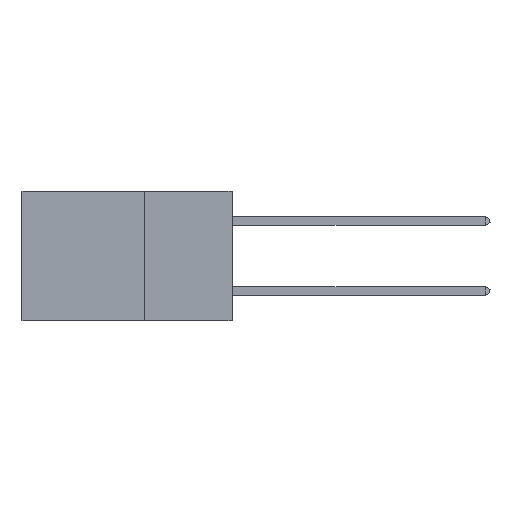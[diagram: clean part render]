
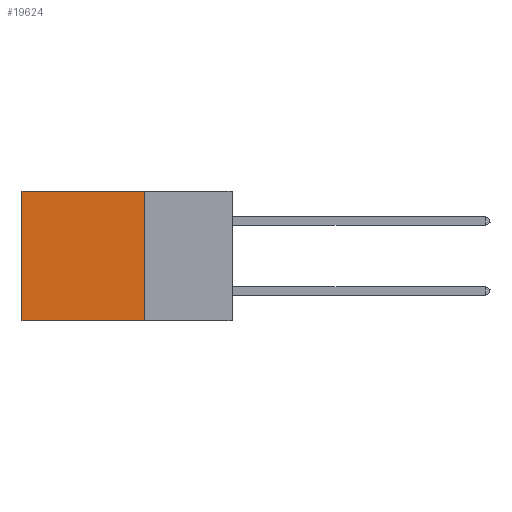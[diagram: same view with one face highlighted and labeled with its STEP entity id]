
A CAD part, left-side view. The second image highlights one B-rep face of the part: STEP entity #19624.
In plain terms, the highlighted planar face has unit normal (-1, 0, 0).
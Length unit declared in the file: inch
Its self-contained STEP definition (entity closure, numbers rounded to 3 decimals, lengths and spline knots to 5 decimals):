
#55 = EDGE_CURVE ( 'NONE', #11595, #7281, #10687, .T. ) ;
#1050 = ORIENTED_EDGE ( 'NONE', *, *, #6455, .F. ) ;
#1164 = CARTESIAN_POINT ( 'NONE',  ( 0.2875, 0.25, -0.37 ) ) ;
#1235 = CARTESIAN_POINT ( 'NONE',  ( 0.2875, 0.6, 0. ) ) ;
#1429 = ORIENTED_EDGE ( 'NONE', *, *, #4409, .T. ) ;
#2161 = ORIENTED_EDGE ( 'NONE', *, *, #55, .T. ) ;
#2571 = LINE ( 'NONE', #23844, #16280 ) ;
#2996 = CARTESIAN_POINT ( 'NONE',  ( 0.2875, 0.6, 0. ) ) ;
#3052 = DIRECTION ( 'NONE',  ( 0., 0., -1. ) ) ;
#4409 = EDGE_CURVE ( 'NONE', #7281, #14466, #6045, .T. ) ;
#4713 = DIRECTION ( 'NONE',  ( 0., 0., -1. ) ) ;
#5467 = VERTEX_POINT ( 'NONE', #1164 ) ;
#5556 = LINE ( 'NONE', #22024, #10125 ) ;
#6045 = LINE ( 'NONE', #2996, #20780 ) ;
#6455 = EDGE_CURVE ( 'NONE', #11595, #5467, #2571, .T. ) ;
#7241 = DIRECTION ( 'NONE',  ( 1., 0., 0. ) ) ;
#7281 = VERTEX_POINT ( 'NONE', #1235 ) ;
#8701 = ORIENTED_EDGE ( 'NONE', *, *, #15763, .F. ) ;
#10125 = VECTOR ( 'NONE', #12718, 39.37008 ) ;
#10687 = LINE ( 'NONE', #15584, #15217 ) ;
#11054 = CARTESIAN_POINT ( 'NONE',  ( 0.2875, 0.25, 0. ) ) ;
#11595 = VERTEX_POINT ( 'NONE', #11054 ) ;
#12066 = EDGE_LOOP ( 'NONE', ( #1429, #8701, #1050, #2161 ) ) ;
#12718 = DIRECTION ( 'NONE',  ( 0., 1., 0. ) ) ;
#14466 = VERTEX_POINT ( 'NONE', #19636 ) ;
#15217 = VECTOR ( 'NONE', #23816, 39.37008 ) ;
#15584 = CARTESIAN_POINT ( 'NONE',  ( 0.2875, 0.25, 0. ) ) ;
#15625 = AXIS2_PLACEMENT_3D ( 'NONE', #18751, #7241, #20661 ) ;
#15657 = FACE_OUTER_BOUND ( 'NONE', #12066, .T. ) ;
#15763 = EDGE_CURVE ( 'NONE', #5467, #14466, #5556, .T. ) ;
#16280 = VECTOR ( 'NONE', #4713, 39.37008 ) ;
#18751 = CARTESIAN_POINT ( 'NONE',  ( 0.2875, 0.25, 0. ) ) ;
#19624 = ADVANCED_FACE ( 'NONE', ( #15657 ), #20575, .F. ) ;
#19636 = CARTESIAN_POINT ( 'NONE',  ( 0.2875, 0.6, -0.37 ) ) ;
#20575 = PLANE ( 'NONE',  #15625 ) ;
#20661 = DIRECTION ( 'NONE',  ( 0., 0., -1. ) ) ;
#20780 = VECTOR ( 'NONE', #3052, 39.37008 ) ;
#22024 = CARTESIAN_POINT ( 'NONE',  ( 0.2875, 0.25, -0.37 ) ) ;
#23816 = DIRECTION ( 'NONE',  ( 0., 1., 0. ) ) ;
#23844 = CARTESIAN_POINT ( 'NONE',  ( 0.2875, 0.25, 0. ) ) ;
